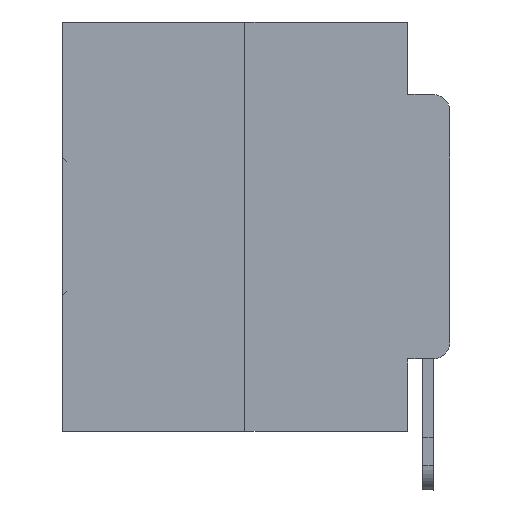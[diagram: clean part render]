
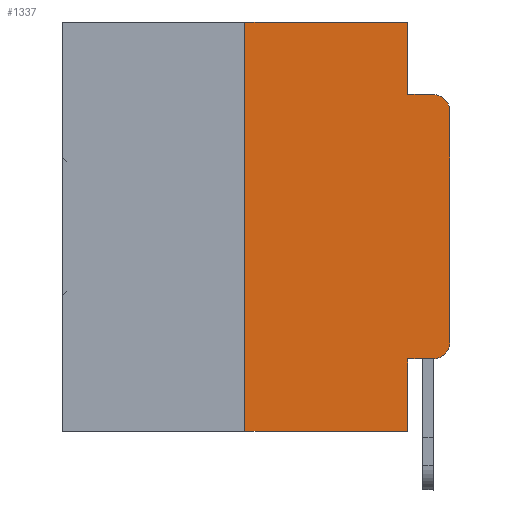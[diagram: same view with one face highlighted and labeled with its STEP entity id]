
A CAD part, left-side view. The second image highlights one B-rep face of the part: STEP entity #1337.
In plain terms, the highlighted planar face has unit normal (-1, 0, 0).
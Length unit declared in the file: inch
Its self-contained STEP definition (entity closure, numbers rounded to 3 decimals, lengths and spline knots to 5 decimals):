
#220 = DIRECTION ( 'NONE',  ( 0., -1., 0. ) ) ;
#349 = ORIENTED_EDGE ( 'NONE', *, *, #21323, .T. ) ;
#783 = VERTEX_POINT ( 'NONE', #6840 ) ;
#1337 = ADVANCED_FACE ( 'NONE', ( #20155 ), #29851, .F. ) ;
#1376 = DIRECTION ( 'NONE',  ( 0., 0., -1. ) ) ;
#1425 = DIRECTION ( 'NONE',  ( -1., 0., 0. ) ) ;
#2038 = ORIENTED_EDGE ( 'NONE', *, *, #14422, .F. ) ;
#2511 = CARTESIAN_POINT ( 'NONE',  ( 0., 0.051, -0.0885 ) ) ;
#2763 = DIRECTION ( 'NONE',  ( 0., 0., -1. ) ) ;
#2829 = LINE ( 'NONE', #24426, #7538 ) ;
#3321 = EDGE_CURVE ( 'NONE', #14130, #13280, #12186, .T. ) ;
#4374 = CARTESIAN_POINT ( 'NONE',  ( 0., 0.051, -0.4115 ) ) ;
#5054 = CARTESIAN_POINT ( 'NONE',  ( 0., 0.25, 0. ) ) ;
#5920 = VECTOR ( 'NONE', #16065, 39.37008 ) ;
#6167 = CARTESIAN_POINT ( 'NONE',  ( 0., 0., -0.1085 ) ) ;
#6744 = LINE ( 'NONE', #16574, #29074 ) ;
#6840 = CARTESIAN_POINT ( 'NONE',  ( 0., 0.02, -0.4115 ) ) ;
#7266 = VERTEX_POINT ( 'NONE', #6167 ) ;
#7280 = EDGE_CURVE ( 'NONE', #19928, #7266, #18574, .T. ) ;
#7538 = VECTOR ( 'NONE', #26987, 39.37008 ) ;
#7542 = ORIENTED_EDGE ( 'NONE', *, *, #7280, .T. ) ;
#7597 = DIRECTION ( 'NONE',  ( 0., 0., -1. ) ) ;
#7638 = EDGE_CURVE ( 'NONE', #7266, #30672, #22628, .T. ) ;
#7732 = ORIENTED_EDGE ( 'NONE', *, *, #16702, .F. ) ;
#8075 = CARTESIAN_POINT ( 'NONE',  ( 0., 0.473, 0. ) ) ;
#8828 = VERTEX_POINT ( 'NONE', #5054 ) ;
#9304 = DIRECTION ( 'NONE',  ( 0., 0., -1. ) ) ;
#9426 = VECTOR ( 'NONE', #220, 39.37008 ) ;
#9756 = CIRCLE ( 'NONE', #29316, 0.02 ) ;
#10326 = CARTESIAN_POINT ( 'NONE',  ( 0., 0.02, -0.3915 ) ) ;
#10515 = VERTEX_POINT ( 'NONE', #4374 ) ;
#11480 = CARTESIAN_POINT ( 'NONE',  ( 0., 0.051, 0. ) ) ;
#11767 = VERTEX_POINT ( 'NONE', #21639 ) ;
#12186 = LINE ( 'NONE', #31397, #20073 ) ;
#12315 = ORIENTED_EDGE ( 'NONE', *, *, #3321, .F. ) ;
#12367 = CARTESIAN_POINT ( 'NONE',  ( 0., 0.051, 0. ) ) ;
#12426 = LINE ( 'NONE', #17112, #9426 ) ;
#13280 = VERTEX_POINT ( 'NONE', #2511 ) ;
#13949 = LINE ( 'NONE', #23786, #5920 ) ;
#14130 = VERTEX_POINT ( 'NONE', #12367 ) ;
#14422 = EDGE_CURVE ( 'NONE', #8828, #14130, #13949, .T. ) ;
#14572 = ORIENTED_EDGE ( 'NONE', *, *, #26541, .F. ) ;
#15990 = CARTESIAN_POINT ( 'NONE',  ( 0., 0., 0. ) ) ;
#16065 = DIRECTION ( 'NONE',  ( 0., -1., 0. ) ) ;
#16259 = CARTESIAN_POINT ( 'NONE',  ( 0., 0., -0.3915 ) ) ;
#16574 = CARTESIAN_POINT ( 'NONE',  ( 0., 0.25, 0. ) ) ;
#16702 = EDGE_CURVE ( 'NONE', #13280, #30672, #2829, .T. ) ;
#16793 = CARTESIAN_POINT ( 'NONE',  ( 0., 0.473, -0.5 ) ) ;
#16999 = CARTESIAN_POINT ( 'NONE',  ( 0., 0.02, -0.0885 ) ) ;
#17112 = CARTESIAN_POINT ( 'NONE',  ( 0., 0.051, -0.4115 ) ) ;
#17355 = VECTOR ( 'NONE', #28708, 39.37008 ) ;
#17735 = DIRECTION ( 'NONE',  ( 1., 0., 0. ) ) ;
#17821 = AXIS2_PLACEMENT_3D ( 'NONE', #8075, #17735, #7597 ) ;
#18574 = LINE ( 'NONE', #15990, #17355 ) ;
#19829 = DIRECTION ( 'NONE',  ( -1., 0., 0. ) ) ;
#19897 = ORIENTED_EDGE ( 'NONE', *, *, #22466, .T. ) ;
#19928 = VERTEX_POINT ( 'NONE', #16259 ) ;
#20073 = VECTOR ( 'NONE', #9304, 39.37008 ) ;
#20155 = FACE_OUTER_BOUND ( 'NONE', #30917, .T. ) ;
#20848 = LINE ( 'NONE', #11480, #27041 ) ;
#20930 = DIRECTION ( 'NONE',  ( 0., 0., 1. ) ) ;
#20974 = VERTEX_POINT ( 'NONE', #22463 ) ;
#21323 = EDGE_CURVE ( 'NONE', #783, #19928, #9756, .T. ) ;
#21639 = CARTESIAN_POINT ( 'NONE',  ( 0., 0.25, -0.5 ) ) ;
#21795 = DIRECTION ( 'NONE',  ( 0., -1., 0. ) ) ;
#22117 = LINE ( 'NONE', #16793, #29908 ) ;
#22156 = AXIS2_PLACEMENT_3D ( 'NONE', #23326, #1425, #30910 ) ;
#22463 = CARTESIAN_POINT ( 'NONE',  ( 0., 0.051, -0.5 ) ) ;
#22466 = EDGE_CURVE ( 'NONE', #11767, #20974, #22117, .T. ) ;
#22628 = CIRCLE ( 'NONE', #22156, 0.02 ) ;
#23326 = CARTESIAN_POINT ( 'NONE',  ( 0., 0.02, -0.1085 ) ) ;
#23714 = EDGE_CURVE ( 'NONE', #10515, #783, #12426, .T. ) ;
#23786 = CARTESIAN_POINT ( 'NONE',  ( 0., 0.473, 0. ) ) ;
#24426 = CARTESIAN_POINT ( 'NONE',  ( 0., 0.051, -0.0885 ) ) ;
#25634 = EDGE_CURVE ( 'NONE', #11767, #8828, #6744, .T. ) ;
#26499 = ORIENTED_EDGE ( 'NONE', *, *, #23714, .T. ) ;
#26541 = EDGE_CURVE ( 'NONE', #10515, #20974, #20848, .T. ) ;
#26987 = DIRECTION ( 'NONE',  ( 0., -1., 0. ) ) ;
#27041 = VECTOR ( 'NONE', #1376, 39.37008 ) ;
#27467 = ORIENTED_EDGE ( 'NONE', *, *, #25634, .F. ) ;
#28708 = DIRECTION ( 'NONE',  ( 0., 0., 1. ) ) ;
#29074 = VECTOR ( 'NONE', #20930, 39.37008 ) ;
#29316 = AXIS2_PLACEMENT_3D ( 'NONE', #10326, #19829, #2763 ) ;
#29851 = PLANE ( 'NONE',  #17821 ) ;
#29908 = VECTOR ( 'NONE', #21795, 39.37008 ) ;
#30672 = VERTEX_POINT ( 'NONE', #16999 ) ;
#30694 = ORIENTED_EDGE ( 'NONE', *, *, #7638, .T. ) ;
#30910 = DIRECTION ( 'NONE',  ( 0., 0., -1. ) ) ;
#30917 = EDGE_LOOP ( 'NONE', ( #7542, #30694, #7732, #12315, #2038, #27467, #19897, #14572, #26499, #349 ) ) ;
#31397 = CARTESIAN_POINT ( 'NONE',  ( 0., 0.051, 0. ) ) ;
